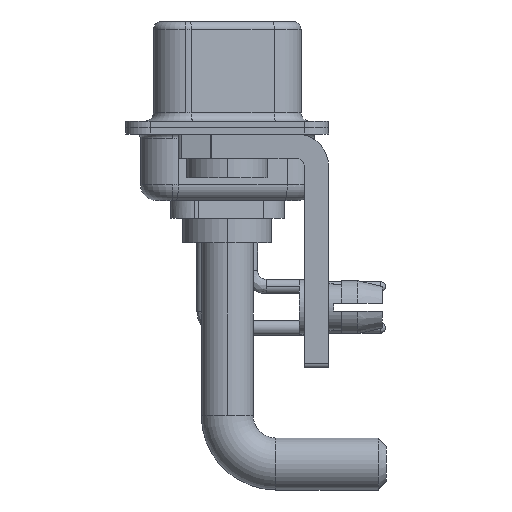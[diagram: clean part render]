
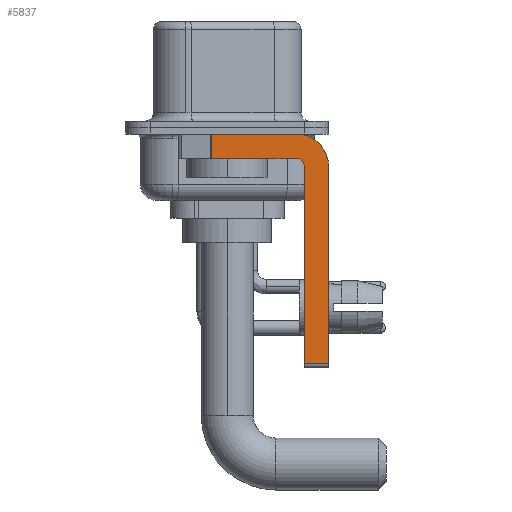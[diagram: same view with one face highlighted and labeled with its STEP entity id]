
A CAD part, left-side view. The second image highlights one B-rep face of the part: STEP entity #5837.
In plain terms, the highlighted planar face has unit normal (-1, 0, 0).
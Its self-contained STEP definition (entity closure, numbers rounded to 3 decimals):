
#364 = EDGE_CURVE ( 'NONE', #12074, #1283, #5236, .T. ) ;
#508 = CARTESIAN_POINT ( 'NONE',  ( -2.9, -4.75, -14.8 ) ) ;
#610 = ORIENTED_EDGE ( 'NONE', *, *, #22845, .F. ) ;
#855 = CARTESIAN_POINT ( 'NONE',  ( -2.9, -4.25, -2.4 ) ) ;
#1283 = VERTEX_POINT ( 'NONE', #17914 ) ;
#1723 = VERTEX_POINT ( 'NONE', #12939 ) ;
#2345 = LINE ( 'NONE', #22903, #9530 ) ;
#2361 = CARTESIAN_POINT ( 'NONE',  ( -2.9, -4.25, -2.4 ) ) ;
#2459 = ORIENTED_EDGE ( 'NONE', *, *, #25196, .T. ) ;
#2568 = DIRECTION ( 'NONE',  ( 0., 0., 1. ) ) ;
#2907 = VECTOR ( 'NONE', #3287, 1000. ) ;
#2972 = VERTEX_POINT ( 'NONE', #7996 ) ;
#3145 = CARTESIAN_POINT ( 'NONE',  ( -2.9, -4.25, -1.9 ) ) ;
#3287 = DIRECTION ( 'NONE',  ( 0., 1., 0. ) ) ;
#3534 = ORIENTED_EDGE ( 'NONE', *, *, #5766, .F. ) ;
#4010 = DIRECTION ( 'NONE',  ( 0., 0., 1. ) ) ;
#4019 = AXIS2_PLACEMENT_3D ( 'NONE', #2361, #18949, #4010 ) ;
#4432 = VECTOR ( 'NONE', #11183, 1000. ) ;
#4555 = PLANE ( 'NONE',  #8107 ) ;
#4936 = LINE ( 'NONE', #3145, #2907 ) ;
#5236 = LINE ( 'NONE', #17575, #17370 ) ;
#5569 = ORIENTED_EDGE ( 'NONE', *, *, #364, .F. ) ;
#5629 = EDGE_LOOP ( 'NONE', ( #14949, #19160, #610, #5890, #6572, #2459, #5569, #3534 ) ) ;
#5766 = EDGE_CURVE ( 'NONE', #23341, #12074, #9417, .T. ) ;
#5837 = ADVANCED_FACE ( 'NONE', ( #19102 ), #4555, .F. ) ;
#5890 = ORIENTED_EDGE ( 'NONE', *, *, #14202, .F. ) ;
#5898 = LINE ( 'NONE', #13825, #10448 ) ;
#6487 = DIRECTION ( 'NONE',  ( 0., 0., -1. ) ) ;
#6572 = ORIENTED_EDGE ( 'NONE', *, *, #12111, .F. ) ;
#6946 = CARTESIAN_POINT ( 'NONE',  ( -2.9, -6.25, -2.4 ) ) ;
#7301 = DIRECTION ( 'NONE',  ( 0., 0., -1. ) ) ;
#7996 = CARTESIAN_POINT ( 'NONE',  ( -2.9, 0.978, -1.9 ) ) ;
#8107 = AXIS2_PLACEMENT_3D ( 'NONE', #17172, #19504, #6487 ) ;
#8732 = VERTEX_POINT ( 'NONE', #24270 ) ;
#8843 = CIRCLE ( 'NONE', #4019, 0.5 ) ;
#9417 = CIRCLE ( 'NONE', #16853, 2. ) ;
#9530 = VECTOR ( 'NONE', #19078, 1000. ) ;
#10448 = VECTOR ( 'NONE', #24521, 1000. ) ;
#11183 = DIRECTION ( 'NONE',  ( 0., -1., 0. ) ) ;
#11259 = DIRECTION ( 'NONE',  ( 0., 0., -1. ) ) ;
#12074 = VERTEX_POINT ( 'NONE', #6946 ) ;
#12111 = EDGE_CURVE ( 'NONE', #21099, #1723, #13219, .T. ) ;
#12939 = CARTESIAN_POINT ( 'NONE',  ( -2.9, -4.75, -2.4 ) ) ;
#13219 = LINE ( 'NONE', #508, #14429 ) ;
#13825 = CARTESIAN_POINT ( 'NONE',  ( -2.9, -4.25, -14.55 ) ) ;
#14088 = EDGE_CURVE ( 'NONE', #23523, #23341, #16099, .T. ) ;
#14202 = EDGE_CURVE ( 'NONE', #1723, #8732, #8843, .T. ) ;
#14429 = VECTOR ( 'NONE', #2568, 1000. ) ;
#14949 = ORIENTED_EDGE ( 'NONE', *, *, #14088, .F. ) ;
#15437 = CARTESIAN_POINT ( 'NONE',  ( -2.9, 3., -0.4 ) ) ;
#16099 = LINE ( 'NONE', #15437, #4432 ) ;
#16853 = AXIS2_PLACEMENT_3D ( 'NONE', #855, #21298, #11259 ) ;
#17172 = CARTESIAN_POINT ( 'NONE',  ( -2.9, -4.25, -2.4 ) ) ;
#17370 = VECTOR ( 'NONE', #7301, 1000. ) ;
#17514 = CARTESIAN_POINT ( 'NONE',  ( -2.9, 0.978, -0.4 ) ) ;
#17575 = CARTESIAN_POINT ( 'NONE',  ( -2.9, -6.25, -2.4 ) ) ;
#17914 = CARTESIAN_POINT ( 'NONE',  ( -2.9, -6.25, -14.55 ) ) ;
#18949 = DIRECTION ( 'NONE',  ( -1., 0., 0. ) ) ;
#19078 = DIRECTION ( 'NONE',  ( 0., 0., -1. ) ) ;
#19102 = FACE_OUTER_BOUND ( 'NONE', #5629, .T. ) ;
#19160 = ORIENTED_EDGE ( 'NONE', *, *, #23582, .T. ) ;
#19504 = DIRECTION ( 'NONE',  ( 1., 0., 0. ) ) ;
#21099 = VERTEX_POINT ( 'NONE', #25250 ) ;
#21298 = DIRECTION ( 'NONE',  ( 1., 0., 0. ) ) ;
#22845 = EDGE_CURVE ( 'NONE', #8732, #2972, #4936, .T. ) ;
#22903 = CARTESIAN_POINT ( 'NONE',  ( -2.9, 0.978, -1.9 ) ) ;
#23341 = VERTEX_POINT ( 'NONE', #25375 ) ;
#23523 = VERTEX_POINT ( 'NONE', #17514 ) ;
#23582 = EDGE_CURVE ( 'NONE', #23523, #2972, #2345, .T. ) ;
#24270 = CARTESIAN_POINT ( 'NONE',  ( -2.9, -4.25, -1.9 ) ) ;
#24521 = DIRECTION ( 'NONE',  ( 0., -1., 0. ) ) ;
#25196 = EDGE_CURVE ( 'NONE', #21099, #1283, #5898, .T. ) ;
#25250 = CARTESIAN_POINT ( 'NONE',  ( -2.9, -4.75, -14.55 ) ) ;
#25375 = CARTESIAN_POINT ( 'NONE',  ( -2.9, -4.25, -0.4 ) ) ;
